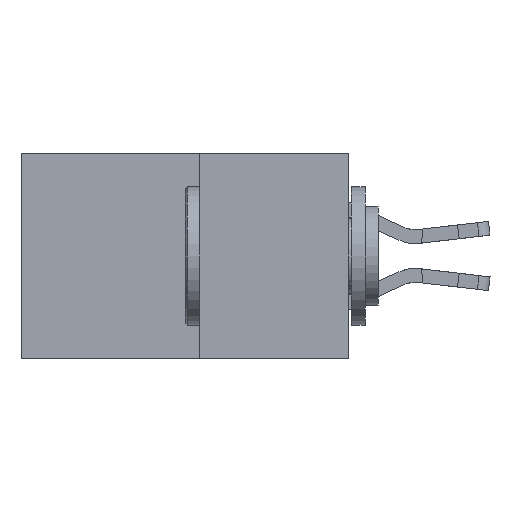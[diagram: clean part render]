
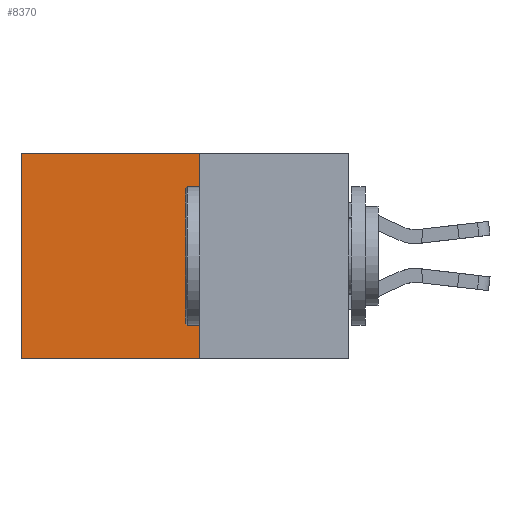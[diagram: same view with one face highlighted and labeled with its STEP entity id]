
A CAD part, left-side view. The second image highlights one B-rep face of the part: STEP entity #8370.
In plain terms, the highlighted planar face has unit normal (-1, 0, 0).
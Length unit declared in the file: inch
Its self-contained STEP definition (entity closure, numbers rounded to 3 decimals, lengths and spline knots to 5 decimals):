
#395 = ORIENTED_EDGE ( 'NONE', *, *, #11962, .T. ) ;
#776 = CARTESIAN_POINT ( 'NONE',  ( 0.277, 0.59, -0.37 ) ) ;
#1027 = EDGE_CURVE ( 'NONE', #7974, #14462, #3196, .T. ) ;
#1903 = ORIENTED_EDGE ( 'NONE', *, *, #5741, .F. ) ;
#1941 = EDGE_CURVE ( 'NONE', #7974, #4325, #15599, .T. ) ;
#2380 = VECTOR ( 'NONE', #14238, 39.37008 ) ;
#2816 = ORIENTED_EDGE ( 'NONE', *, *, #1941, .F. ) ;
#3196 = LINE ( 'NONE', #12714, #5767 ) ;
#3669 = VECTOR ( 'NONE', #14026, 39.37008 ) ;
#3864 = DIRECTION ( 'NONE',  ( 0., 1., 0. ) ) ;
#4325 = VERTEX_POINT ( 'NONE', #5399 ) ;
#4872 = ORIENTED_EDGE ( 'NONE', *, *, #1027, .T. ) ;
#4942 = CARTESIAN_POINT ( 'NONE',  ( 0.277, 0.27, -0.37 ) ) ;
#5261 = DIRECTION ( 'NONE',  ( 1., 0., 0. ) ) ;
#5307 = CARTESIAN_POINT ( 'NONE',  ( 0.277, 0.59, -0.37 ) ) ;
#5399 = CARTESIAN_POINT ( 'NONE',  ( 0.277, 0.27, -0.37 ) ) ;
#5741 = EDGE_CURVE ( 'NONE', #4325, #5978, #8307, .T. ) ;
#5767 = VECTOR ( 'NONE', #3864, 39.37008 ) ;
#5978 = VERTEX_POINT ( 'NONE', #776 ) ;
#6452 = CARTESIAN_POINT ( 'NONE',  ( 0.277, 0.27, -0.37 ) ) ;
#6830 = DIRECTION ( 'NONE',  ( 0., 1., 0. ) ) ;
#6978 = CARTESIAN_POINT ( 'NONE',  ( 0.277, 0.27, -0.37 ) ) ;
#7916 = VECTOR ( 'NONE', #6830, 39.37008 ) ;
#7974 = VERTEX_POINT ( 'NONE', #10674 ) ;
#8307 = LINE ( 'NONE', #6978, #7916 ) ;
#8370 = ADVANCED_FACE ( 'NONE', ( #11944 ), #12662, .F. ) ;
#8449 = AXIS2_PLACEMENT_3D ( 'NONE', #6452, #5261, #13921 ) ;
#9943 = CARTESIAN_POINT ( 'NONE',  ( 0.277, 0.59, 0. ) ) ;
#10674 = CARTESIAN_POINT ( 'NONE',  ( 0.277, 0.27, 0. ) ) ;
#11944 = FACE_OUTER_BOUND ( 'NONE', #12301, .T. ) ;
#11962 = EDGE_CURVE ( 'NONE', #14462, #5978, #13991, .T. ) ;
#12301 = EDGE_LOOP ( 'NONE', ( #395, #1903, #2816, #4872 ) ) ;
#12662 = PLANE ( 'NONE',  #8449 ) ;
#12714 = CARTESIAN_POINT ( 'NONE',  ( 0.277, 0.27, 0. ) ) ;
#13921 = DIRECTION ( 'NONE',  ( 0., 0., -1. ) ) ;
#13991 = LINE ( 'NONE', #5307, #3669 ) ;
#14026 = DIRECTION ( 'NONE',  ( 0., 0., -1. ) ) ;
#14238 = DIRECTION ( 'NONE',  ( 0., 0., -1. ) ) ;
#14462 = VERTEX_POINT ( 'NONE', #9943 ) ;
#15599 = LINE ( 'NONE', #4942, #2380 ) ;
